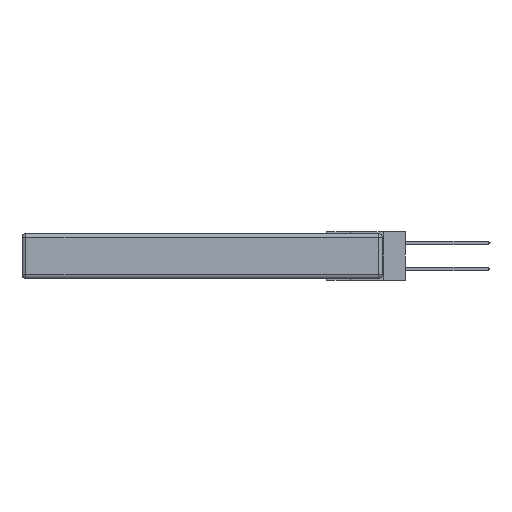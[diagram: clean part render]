
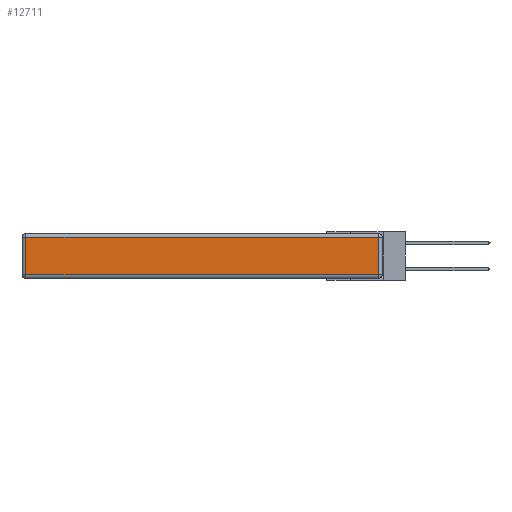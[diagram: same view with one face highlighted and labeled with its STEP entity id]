
A CAD part, left-side view. The second image highlights one B-rep face of the part: STEP entity #12711.
In plain terms, the highlighted planar face has unit normal (-1, 0, 0).
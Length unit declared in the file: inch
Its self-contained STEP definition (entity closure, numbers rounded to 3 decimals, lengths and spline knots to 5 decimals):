
#17 = FACE_OUTER_BOUND ( 'NONE', #11337, .T. ) ;
#617 = DIRECTION ( 'NONE',  ( 0., -1., 0. ) ) ;
#3595 = DIRECTION ( 'NONE',  ( 0., 1., 0. ) ) ;
#4038 = ORIENTED_EDGE ( 'NONE', *, *, #18672, .T. ) ;
#4988 = CARTESIAN_POINT ( 'NONE',  ( 0., 0.03, -0.313 ) ) ;
#6196 = CARTESIAN_POINT ( 'NONE',  ( 0., 0., -0.343 ) ) ;
#6759 = LINE ( 'NONE', #9226, #15325 ) ;
#7140 = ORIENTED_EDGE ( 'NONE', *, *, #23804, .T. ) ;
#7166 = DIRECTION ( 'NONE',  ( 0., 0., 1. ) ) ;
#8390 = DIRECTION ( 'NONE',  ( 0., 0., 1. ) ) ;
#9226 = CARTESIAN_POINT ( 'NONE',  ( 0., 2.72, -0.343 ) ) ;
#11337 = EDGE_LOOP ( 'NONE', ( #19585, #4038, #7140, #21814 ) ) ;
#11520 = VECTOR ( 'NONE', #7166, 39.37008 ) ;
#11809 = CARTESIAN_POINT ( 'NONE',  ( 0., 2.72, -0.03 ) ) ;
#12172 = VERTEX_POINT ( 'NONE', #4988 ) ;
#12711 = ADVANCED_FACE ( 'NONE', ( #17 ), #14904, .T. ) ;
#13303 = CARTESIAN_POINT ( 'NONE',  ( 0., 0.03, -0.03 ) ) ;
#13768 = CARTESIAN_POINT ( 'NONE',  ( 0., 0.03, -0.343 ) ) ;
#14004 = EDGE_CURVE ( 'NONE', #19416, #20625, #6759, .T. ) ;
#14904 = PLANE ( 'NONE',  #21714 ) ;
#15325 = VECTOR ( 'NONE', #22470, 39.37008 ) ;
#15768 = VECTOR ( 'NONE', #617, 39.37008 ) ;
#16328 = LINE ( 'NONE', #13768, #11520 ) ;
#18672 = EDGE_CURVE ( 'NONE', #12172, #27369, #16328, .T. ) ;
#19416 = VERTEX_POINT ( 'NONE', #11809 ) ;
#19585 = ORIENTED_EDGE ( 'NONE', *, *, #25008, .T. ) ;
#20625 = VERTEX_POINT ( 'NONE', #22957 ) ;
#21465 = DIRECTION ( 'NONE',  ( -1., 0., 0. ) ) ;
#21714 = AXIS2_PLACEMENT_3D ( 'NONE', #6196, #21465, #8390 ) ;
#21814 = ORIENTED_EDGE ( 'NONE', *, *, #14004, .T. ) ;
#21967 = LINE ( 'NONE', #27330, #22632 ) ;
#22470 = DIRECTION ( 'NONE',  ( 0., 0., -1. ) ) ;
#22583 = LINE ( 'NONE', #26461, #15768 ) ;
#22632 = VECTOR ( 'NONE', #3595, 39.37008 ) ;
#22957 = CARTESIAN_POINT ( 'NONE',  ( 0., 2.72, -0.313 ) ) ;
#23804 = EDGE_CURVE ( 'NONE', #27369, #19416, #21967, .T. ) ;
#25008 = EDGE_CURVE ( 'NONE', #20625, #12172, #22583, .T. ) ;
#26461 = CARTESIAN_POINT ( 'NONE',  ( 0., 0., -0.313 ) ) ;
#27330 = CARTESIAN_POINT ( 'NONE',  ( 0., 2.75, -0.03 ) ) ;
#27369 = VERTEX_POINT ( 'NONE', #13303 ) ;
